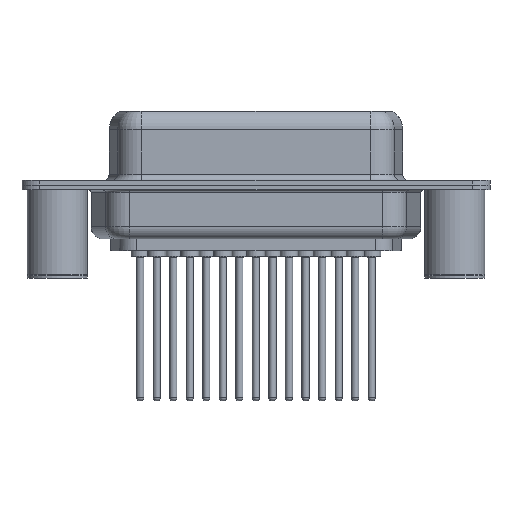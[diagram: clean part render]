
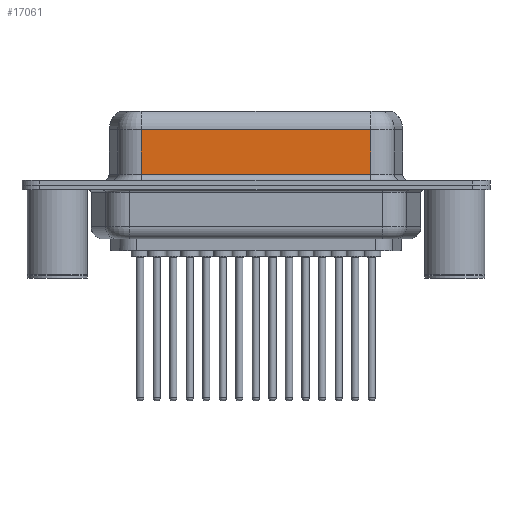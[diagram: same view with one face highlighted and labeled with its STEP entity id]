
A CAD part, front view. The second image highlights one B-rep face of the part: STEP entity #17061.
In plain terms, the highlighted planar face has unit normal (0, -1, 0).
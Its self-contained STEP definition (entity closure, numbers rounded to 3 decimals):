
#933 = VERTEX_POINT ( 'NONE', #10960 ) ;
#937 = VERTEX_POINT ( 'NONE', #12282 ) ;
#1463 = VECTOR ( 'NONE', #8812, 1000. ) ;
#2303 = EDGE_CURVE ( 'NONE', #10449, #937, #12715, .T. ) ;
#2504 = CARTESIAN_POINT ( 'NONE',  ( 26.262, -3.95, 6.4 ) ) ;
#2705 = VECTOR ( 'NONE', #11204, 1000. ) ;
#2901 = LINE ( 'NONE', #13036, #6927 ) ;
#4018 = FACE_OUTER_BOUND ( 'NONE', #17640, .T. ) ;
#4493 = DIRECTION ( 'NONE',  ( 1., 0., 0. ) ) ;
#5241 = DIRECTION ( 'NONE',  ( 0., 1., 0. ) ) ;
#5348 = EDGE_CURVE ( 'NONE', #933, #16426, #17732, .T. ) ;
#5734 = LINE ( 'NONE', #9964, #1463 ) ;
#6056 = DIRECTION ( 'NONE',  ( 0., 0., -1. ) ) ;
#6427 = CARTESIAN_POINT ( 'NONE',  ( 26.262, -3.95, 6.4 ) ) ;
#6927 = VECTOR ( 'NONE', #4493, 1000. ) ;
#7266 = CARTESIAN_POINT ( 'NONE',  ( 7.038, -3.95, 4.65 ) ) ;
#7366 = EDGE_CURVE ( 'NONE', #937, #16426, #2901, .T. ) ;
#8233 = DIRECTION ( 'NONE',  ( -1., 0., 0. ) ) ;
#8430 = ORIENTED_EDGE ( 'NONE', *, *, #5348, .F. ) ;
#8812 = DIRECTION ( 'NONE',  ( -1., 0., 0. ) ) ;
#9236 = VECTOR ( 'NONE', #6056, 1000. ) ;
#9375 = PLANE ( 'NONE',  #9527 ) ;
#9527 = AXIS2_PLACEMENT_3D ( 'NONE', #2504, #5241, #8233 ) ;
#9964 = CARTESIAN_POINT ( 'NONE',  ( 26.262, -3.95, 4.65 ) ) ;
#10449 = VERTEX_POINT ( 'NONE', #7266 ) ;
#10926 = CARTESIAN_POINT ( 'NONE',  ( 7.038, -3.95, 6.4 ) ) ;
#10960 = CARTESIAN_POINT ( 'NONE',  ( 26.262, -3.95, 4.65 ) ) ;
#11204 = DIRECTION ( 'NONE',  ( 0., 0., -1. ) ) ;
#12282 = CARTESIAN_POINT ( 'NONE',  ( 7.038, -3.95, 0.9 ) ) ;
#12590 = EDGE_CURVE ( 'NONE', #933, #10449, #5734, .T. ) ;
#12715 = LINE ( 'NONE', #10926, #2705 ) ;
#13036 = CARTESIAN_POINT ( 'NONE',  ( 26.262, -3.95, 0.9 ) ) ;
#14084 = CARTESIAN_POINT ( 'NONE',  ( 26.262, -3.95, 0.9 ) ) ;
#15905 = ORIENTED_EDGE ( 'NONE', *, *, #7366, .T. ) ;
#15946 = ORIENTED_EDGE ( 'NONE', *, *, #2303, .T. ) ;
#16426 = VERTEX_POINT ( 'NONE', #14084 ) ;
#17061 = ADVANCED_FACE ( 'NONE', ( #4018 ), #9375, .F. ) ;
#17640 = EDGE_LOOP ( 'NONE', ( #8430, #18164, #15946, #15905 ) ) ;
#17732 = LINE ( 'NONE', #6427, #9236 ) ;
#18164 = ORIENTED_EDGE ( 'NONE', *, *, #12590, .T. ) ;
